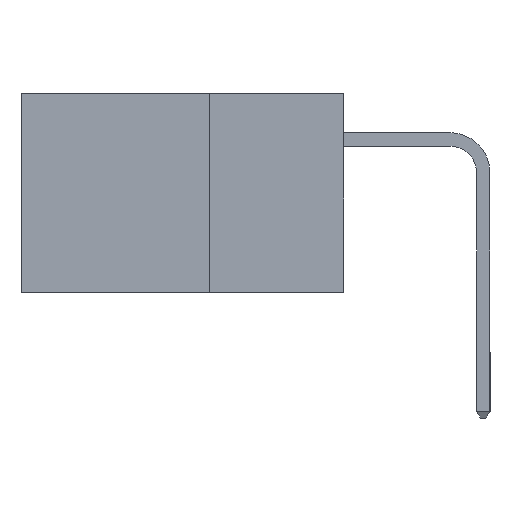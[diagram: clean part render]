
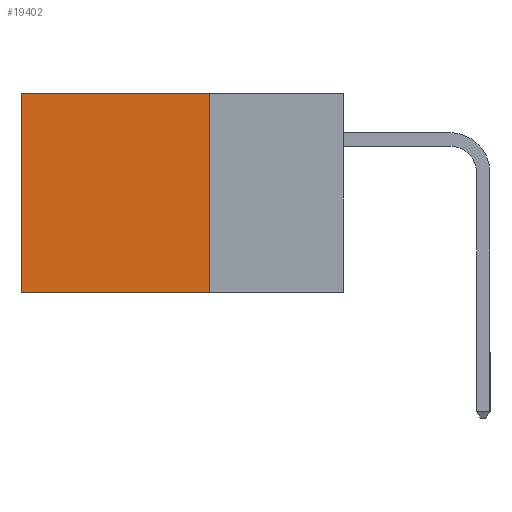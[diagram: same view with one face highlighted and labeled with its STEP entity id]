
A CAD part, left-side view. The second image highlights one B-rep face of the part: STEP entity #19402.
In plain terms, the highlighted planar face has unit normal (-1, 0, 0).
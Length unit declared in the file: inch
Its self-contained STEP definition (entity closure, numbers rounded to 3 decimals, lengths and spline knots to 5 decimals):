
#795 = VERTEX_POINT ( 'NONE', #12905 ) ;
#900 = VECTOR ( 'NONE', #5135, 39.37008 ) ;
#1291 = ORIENTED_EDGE ( 'NONE', *, *, #19166, .T. ) ;
#1836 = DIRECTION ( 'NONE',  ( 0., 0., -1. ) ) ;
#1930 = DIRECTION ( 'NONE',  ( 0., 1., 0. ) ) ;
#2259 = ORIENTED_EDGE ( 'NONE', *, *, #17752, .F. ) ;
#2384 = ORIENTED_EDGE ( 'NONE', *, *, #4280, .F. ) ;
#3118 = VECTOR ( 'NONE', #19372, 39.37008 ) ;
#3389 = CARTESIAN_POINT ( 'NONE',  ( 0.298, 0.25, 0. ) ) ;
#4083 = DIRECTION ( 'NONE',  ( 0., 0., -1. ) ) ;
#4280 = EDGE_CURVE ( 'NONE', #13121, #12729, #8514, .T. ) ;
#5084 = LINE ( 'NONE', #8277, #900 ) ;
#5135 = DIRECTION ( 'NONE',  ( 0., 1., 0. ) ) ;
#5587 = CARTESIAN_POINT ( 'NONE',  ( 0.298, 0.25, 0. ) ) ;
#6514 = CARTESIAN_POINT ( 'NONE',  ( 0.298, 0.25, -0.37 ) ) ;
#6576 = CARTESIAN_POINT ( 'NONE',  ( 0.298, 0.6, -0.37 ) ) ;
#8277 = CARTESIAN_POINT ( 'NONE',  ( 0.298, 0.25, 0. ) ) ;
#8514 = LINE ( 'NONE', #19115, #9001 ) ;
#9001 = VECTOR ( 'NONE', #1930, 39.37008 ) ;
#11502 = LINE ( 'NONE', #17836, #3118 ) ;
#11947 = PLANE ( 'NONE',  #17064 ) ;
#12246 = ORIENTED_EDGE ( 'NONE', *, *, #19275, .T. ) ;
#12411 = EDGE_LOOP ( 'NONE', ( #12246, #2384, #2259, #1291 ) ) ;
#12729 = VERTEX_POINT ( 'NONE', #6576 ) ;
#12905 = CARTESIAN_POINT ( 'NONE',  ( 0.298, 0.25, 0. ) ) ;
#13121 = VERTEX_POINT ( 'NONE', #6514 ) ;
#13468 = DIRECTION ( 'NONE',  ( 1., 0., 0. ) ) ;
#14834 = VERTEX_POINT ( 'NONE', #18562 ) ;
#16887 = VECTOR ( 'NONE', #1836, 39.37008 ) ;
#17064 = AXIS2_PLACEMENT_3D ( 'NONE', #5587, #13468, #4083 ) ;
#17304 = FACE_OUTER_BOUND ( 'NONE', #12411, .T. ) ;
#17392 = LINE ( 'NONE', #3389, #16887 ) ;
#17752 = EDGE_CURVE ( 'NONE', #795, #13121, #17392, .T. ) ;
#17836 = CARTESIAN_POINT ( 'NONE',  ( 0.298, 0.6, 0. ) ) ;
#18562 = CARTESIAN_POINT ( 'NONE',  ( 0.298, 0.6, 0. ) ) ;
#19115 = CARTESIAN_POINT ( 'NONE',  ( 0.298, 0.25, -0.37 ) ) ;
#19166 = EDGE_CURVE ( 'NONE', #795, #14834, #5084, .T. ) ;
#19275 = EDGE_CURVE ( 'NONE', #14834, #12729, #11502, .T. ) ;
#19372 = DIRECTION ( 'NONE',  ( 0., 0., -1. ) ) ;
#19402 = ADVANCED_FACE ( 'NONE', ( #17304 ), #11947, .F. ) ;
